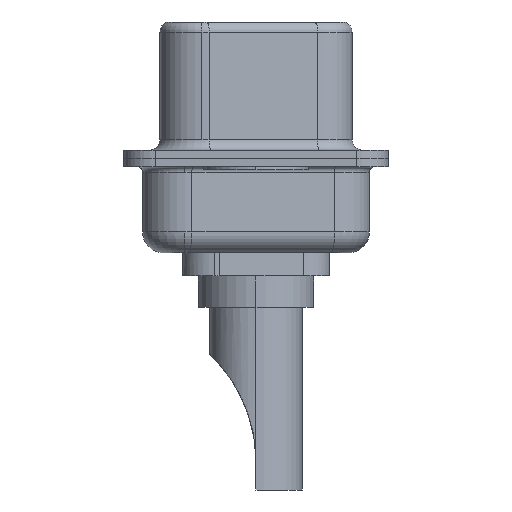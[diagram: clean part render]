
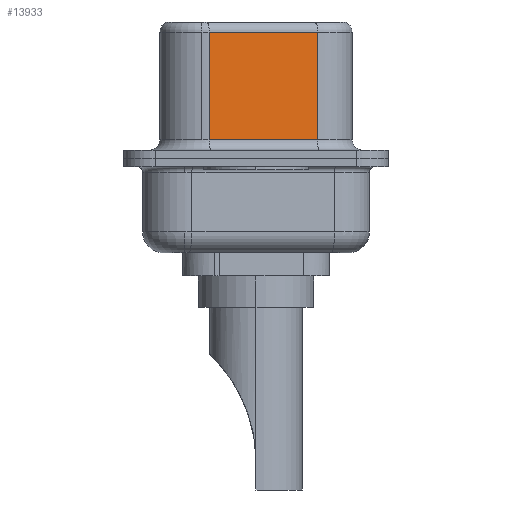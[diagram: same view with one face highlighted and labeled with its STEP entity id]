
A CAD part, left-side view. The second image highlights one B-rep face of the part: STEP entity #13933.
In plain terms, the highlighted planar face has unit normal (-0.985, -0.174, 0).
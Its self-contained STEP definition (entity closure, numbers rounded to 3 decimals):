
#855 = VECTOR ( 'NONE', #6982, 1000. ) ;
#985 = AXIS2_PLACEMENT_3D ( 'NONE', #8630, #2160, #3576 ) ;
#1518 = CARTESIAN_POINT ( 'NONE',  ( 4.585, -2.927, 0.9 ) ) ;
#1747 = FACE_OUTER_BOUND ( 'NONE', #3736, .T. ) ;
#1927 = CARTESIAN_POINT ( 'NONE',  ( 4.585, -2.927, 0.9 ) ) ;
#1928 = ORIENTED_EDGE ( 'NONE', *, *, #5612, .T. ) ;
#2026 = VECTOR ( 'NONE', #15486, 1000. ) ;
#2160 = DIRECTION ( 'NONE',  ( 0.985, 0.174, 0. ) ) ;
#2650 = CARTESIAN_POINT ( 'NONE',  ( 4.585, -2.927, 6.02 ) ) ;
#2787 = LINE ( 'NONE', #15641, #9653 ) ;
#3172 = ORIENTED_EDGE ( 'NONE', *, *, #12629, .T. ) ;
#3244 = LINE ( 'NONE', #1927, #13081 ) ;
#3576 = DIRECTION ( 'NONE',  ( -0.174, 0.985, 0. ) ) ;
#3736 = EDGE_LOOP ( 'NONE', ( #5828, #1928, #11915, #3172 ) ) ;
#5223 = VERTEX_POINT ( 'NONE', #1518 ) ;
#5612 = EDGE_CURVE ( 'NONE', #15237, #10166, #2787, .T. ) ;
#5828 = ORIENTED_EDGE ( 'NONE', *, *, #16072, .F. ) ;
#6982 = DIRECTION ( 'NONE',  ( 0., 0., -1. ) ) ;
#8240 = DIRECTION ( 'NONE',  ( -0.174, 0.985, 0. ) ) ;
#8391 = CARTESIAN_POINT ( 'NONE',  ( 3.675, 2.233, 6.02 ) ) ;
#8630 = CARTESIAN_POINT ( 'NONE',  ( 4.585, -2.927, 6.52 ) ) ;
#9653 = VECTOR ( 'NONE', #8240, 1000. ) ;
#9689 = DIRECTION ( 'NONE',  ( 0.174, -0.985, 0. ) ) ;
#10166 = VERTEX_POINT ( 'NONE', #8391 ) ;
#10539 = EDGE_CURVE ( 'NONE', #10166, #12967, #16164, .T. ) ;
#11291 = PLANE ( 'NONE',  #985 ) ;
#11915 = ORIENTED_EDGE ( 'NONE', *, *, #10539, .T. ) ;
#12100 = CARTESIAN_POINT ( 'NONE',  ( 4.585, -2.927, 6.52 ) ) ;
#12629 = EDGE_CURVE ( 'NONE', #12967, #5223, #3244, .T. ) ;
#12912 = CARTESIAN_POINT ( 'NONE',  ( 3.675, 2.233, 6.52 ) ) ;
#12967 = VERTEX_POINT ( 'NONE', #13136 ) ;
#13081 = VECTOR ( 'NONE', #9689, 1000. ) ;
#13136 = CARTESIAN_POINT ( 'NONE',  ( 3.675, 2.233, 0.9 ) ) ;
#13933 = ADVANCED_FACE ( 'NONE', ( #1747 ), #11291, .F. ) ;
#14156 = LINE ( 'NONE', #12100, #855 ) ;
#15237 = VERTEX_POINT ( 'NONE', #2650 ) ;
#15486 = DIRECTION ( 'NONE',  ( 0., 0., -1. ) ) ;
#15641 = CARTESIAN_POINT ( 'NONE',  ( 4.585, -2.927, 6.02 ) ) ;
#16072 = EDGE_CURVE ( 'NONE', #15237, #5223, #14156, .T. ) ;
#16164 = LINE ( 'NONE', #12912, #2026 ) ;
